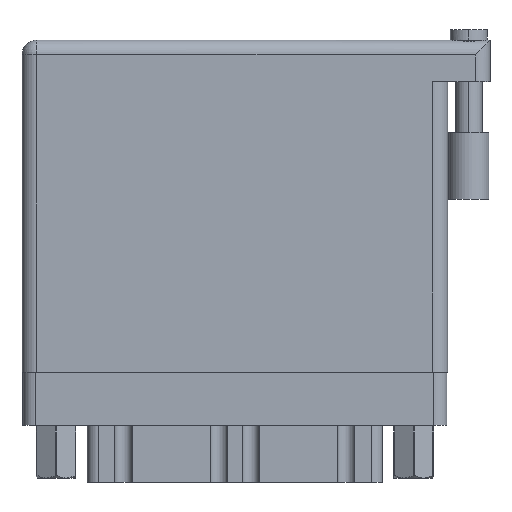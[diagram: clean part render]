
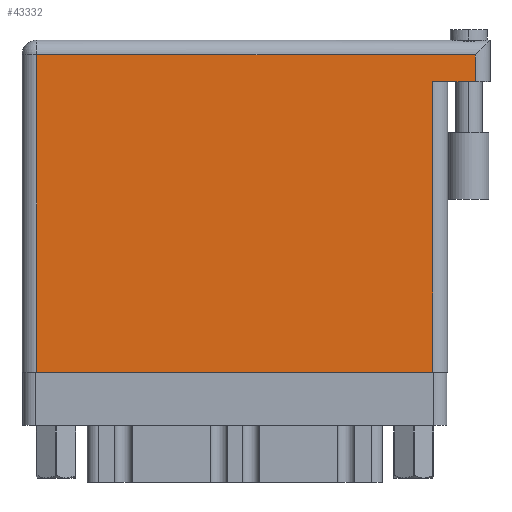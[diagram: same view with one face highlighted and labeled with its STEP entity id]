
A CAD part, front view. The second image highlights one B-rep face of the part: STEP entity #43332.
In plain terms, the highlighted face is planar.
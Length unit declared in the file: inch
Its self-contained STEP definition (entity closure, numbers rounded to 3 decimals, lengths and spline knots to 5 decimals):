
#690 = EDGE_CURVE ( 'NONE', #26756, #20534, #27365, .T. ) ;
#1245 = AXIS2_PLACEMENT_3D ( 'NONE', #22565, #15908, #26881 ) ;
#1280 = VECTOR ( 'NONE', #45791, 39.37008 ) ;
#1360 = PLANE ( 'NONE',  #1245 ) ;
#1695 = VERTEX_POINT ( 'NONE', #16511 ) ;
#1850 = CARTESIAN_POINT ( 'NONE',  ( 2.138, 1.566, 0. ) ) ;
#4083 = CARTESIAN_POINT ( 'NONE',  ( 2.138, 1.369, 0. ) ) ;
#5263 = VECTOR ( 'NONE', #19716, 39.37008 ) ;
#5719 = CARTESIAN_POINT ( 'NONE',  ( 0., 0., 0. ) ) ;
#7614 = ORIENTED_EDGE ( 'NONE', *, *, #45025, .T. ) ;
#8206 = VECTOR ( 'NONE', #32954, 39.37008 ) ;
#8967 = VECTOR ( 'NONE', #31943, 39.37008 ) ;
#11615 = ORIENTED_EDGE ( 'NONE', *, *, #26547, .T. ) ;
#14579 = ORIENTED_EDGE ( 'NONE', *, *, #26457, .T. ) ;
#15660 = EDGE_CURVE ( 'NONE', #26756, #1695, #32720, .T. ) ;
#15908 = DIRECTION ( 'NONE',  ( 0., 0., -1. ) ) ;
#16011 = LINE ( 'NONE', #5719, #1280 ) ;
#16511 = CARTESIAN_POINT ( 'NONE',  ( 1.938, 1.369, 0. ) ) ;
#17248 = CARTESIAN_POINT ( 'NONE',  ( 0.07, 0., 0. ) ) ;
#17375 = LINE ( 'NONE', #20483, #8967 ) ;
#17751 = DIRECTION ( 'NONE',  ( 0., 1., 0. ) ) ;
#19241 = FACE_OUTER_BOUND ( 'NONE', #27735, .T. ) ;
#19716 = DIRECTION ( 'NONE',  ( 0., 1., 0. ) ) ;
#20483 = CARTESIAN_POINT ( 'NONE',  ( 0., 1.496, 0. ) ) ;
#20534 = VERTEX_POINT ( 'NONE', #27502 ) ;
#22565 = CARTESIAN_POINT ( 'NONE',  ( 0., 1.566, 0. ) ) ;
#23859 = ORIENTED_EDGE ( 'NONE', *, *, #690, .T. ) ;
#24574 = VERTEX_POINT ( 'NONE', #25525 ) ;
#25525 = CARTESIAN_POINT ( 'NONE',  ( 0.07, 1.496, 0. ) ) ;
#25597 = LINE ( 'NONE', #32322, #40869 ) ;
#26457 = EDGE_CURVE ( 'NONE', #43823, #1695, #25597, .T. ) ;
#26547 = EDGE_CURVE ( 'NONE', #24574, #38543, #28434, .T. ) ;
#26756 = VERTEX_POINT ( 'NONE', #4083 ) ;
#26879 = EDGE_CURVE ( 'NONE', #38543, #43823, #16011, .T. ) ;
#26881 = DIRECTION ( 'NONE',  ( -1., 0., 0. ) ) ;
#27365 = LINE ( 'NONE', #1850, #5263 ) ;
#27502 = CARTESIAN_POINT ( 'NONE',  ( 2.138, 1.496, 0. ) ) ;
#27735 = EDGE_LOOP ( 'NONE', ( #32025, #14579, #46695, #23859, #7614, #11615 ) ) ;
#28434 = LINE ( 'NONE', #29149, #36309 ) ;
#29149 = CARTESIAN_POINT ( 'NONE',  ( 0.07, 0., 0. ) ) ;
#31943 = DIRECTION ( 'NONE',  ( -1., 0., 0. ) ) ;
#32025 = ORIENTED_EDGE ( 'NONE', *, *, #26879, .T. ) ;
#32322 = CARTESIAN_POINT ( 'NONE',  ( 1.938, 1.369, 0. ) ) ;
#32720 = LINE ( 'NONE', #36517, #8206 ) ;
#32954 = DIRECTION ( 'NONE',  ( -1., 0., 0. ) ) ;
#36309 = VECTOR ( 'NONE', #42980, 39.37008 ) ;
#36517 = CARTESIAN_POINT ( 'NONE',  ( 2.208, 1.369, 0. ) ) ;
#38543 = VERTEX_POINT ( 'NONE', #17248 ) ;
#40869 = VECTOR ( 'NONE', #17751, 39.37008 ) ;
#42305 = CARTESIAN_POINT ( 'NONE',  ( 1.938, 0., 0. ) ) ;
#42980 = DIRECTION ( 'NONE',  ( 0., -1., 0. ) ) ;
#43332 = ADVANCED_FACE ( 'NONE', ( #19241 ), #1360, .F. ) ;
#43823 = VERTEX_POINT ( 'NONE', #42305 ) ;
#45025 = EDGE_CURVE ( 'NONE', #20534, #24574, #17375, .T. ) ;
#45791 = DIRECTION ( 'NONE',  ( 1., 0., 0. ) ) ;
#46695 = ORIENTED_EDGE ( 'NONE', *, *, #15660, .F. ) ;
